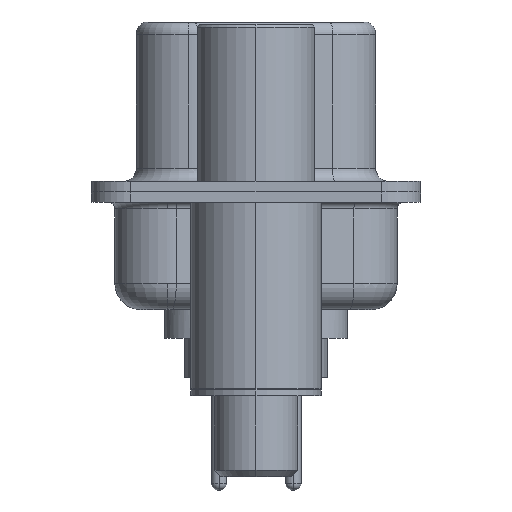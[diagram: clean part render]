
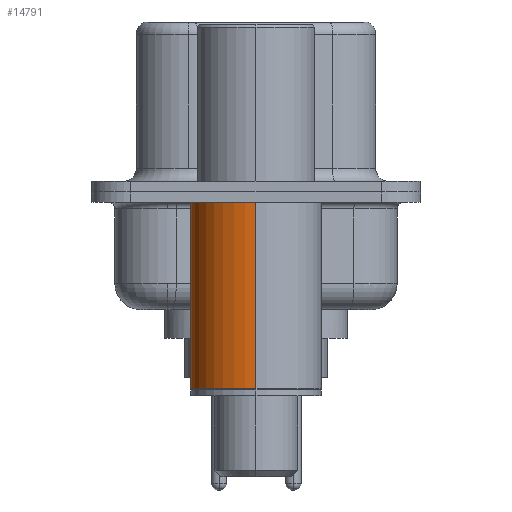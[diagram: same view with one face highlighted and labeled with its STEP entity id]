
A CAD part, left-side view. The second image highlights one B-rep face of the part: STEP entity #14791.
In plain terms, the highlighted cylindrical face has radius 2.5 mm (diameter 5 mm), a partial arc.
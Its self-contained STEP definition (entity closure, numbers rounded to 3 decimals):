
#1159 = EDGE_CURVE ( 'NONE', #7783, #21015, #15888, .T. ) ;
#2001 = DIRECTION ( 'NONE',  ( 0., 0., 1. ) ) ;
#2434 = AXIS2_PLACEMENT_3D ( 'NONE', #13179, #2001, #15097 ) ;
#7620 = DIRECTION ( 'NONE',  ( 1., 0., 0. ) ) ;
#7783 = VERTEX_POINT ( 'NONE', #15548 ) ;
#8595 = CARTESIAN_POINT ( 'NONE',  ( -2.5, 0., -0.4 ) ) ;
#8681 = FACE_OUTER_BOUND ( 'NONE', #11398, .T. ) ;
#8783 = EDGE_CURVE ( 'NONE', #21015, #13180, #20556, .T. ) ;
#9570 = EDGE_CURVE ( 'NONE', #12052, #13180, #22918, .T. ) ;
#10222 = ORIENTED_EDGE ( 'NONE', *, *, #8783, .F. ) ;
#10861 = VECTOR ( 'NONE', #14720, 1000. ) ;
#11142 = DIRECTION ( 'NONE',  ( 0., 0., 1. ) ) ;
#11398 = EDGE_LOOP ( 'NONE', ( #20357, #17075, #10222, #19577 ) ) ;
#11399 = CARTESIAN_POINT ( 'NONE',  ( -2.5, 0., -7.525 ) ) ;
#12052 = VERTEX_POINT ( 'NONE', #11399 ) ;
#12962 = VECTOR ( 'NONE', #20549, 1000. ) ;
#13093 = DIRECTION ( 'NONE',  ( 0., 0., 1. ) ) ;
#13179 = CARTESIAN_POINT ( 'NONE',  ( 0., 0., -7.525 ) ) ;
#13180 = VERTEX_POINT ( 'NONE', #8595 ) ;
#14642 = CARTESIAN_POINT ( 'NONE',  ( 2.5, 0., 0.581 ) ) ;
#14720 = DIRECTION ( 'NONE',  ( 0., 0., 1. ) ) ;
#14791 = ADVANCED_FACE ( 'NONE', ( #8681 ), #23015, .T. ) ;
#14832 = AXIS2_PLACEMENT_3D ( 'NONE', #18840, #13093, #7620 ) ;
#15050 = AXIS2_PLACEMENT_3D ( 'NONE', #22352, #11142, #24262 ) ;
#15097 = DIRECTION ( 'NONE',  ( 1., 0., 0. ) ) ;
#15548 = CARTESIAN_POINT ( 'NONE',  ( 2.5, 0., -7.525 ) ) ;
#15888 = LINE ( 'NONE', #14642, #10861 ) ;
#16976 = CARTESIAN_POINT ( 'NONE',  ( -2.5, 0., 0.581 ) ) ;
#17075 = ORIENTED_EDGE ( 'NONE', *, *, #9570, .T. ) ;
#18625 = CIRCLE ( 'NONE', #2434, 2.5 ) ;
#18840 = CARTESIAN_POINT ( 'NONE',  ( 0., 0., 0.581 ) ) ;
#19577 = ORIENTED_EDGE ( 'NONE', *, *, #1159, .F. ) ;
#20357 = ORIENTED_EDGE ( 'NONE', *, *, #23388, .T. ) ;
#20549 = DIRECTION ( 'NONE',  ( 0., 0., 1. ) ) ;
#20556 = CIRCLE ( 'NONE', #15050, 2.5 ) ;
#21015 = VERTEX_POINT ( 'NONE', #23736 ) ;
#22352 = CARTESIAN_POINT ( 'NONE',  ( 0., 0., -0.4 ) ) ;
#22918 = LINE ( 'NONE', #16976, #12962 ) ;
#23015 = CYLINDRICAL_SURFACE ( 'NONE', #14832, 2.5 ) ;
#23388 = EDGE_CURVE ( 'NONE', #7783, #12052, #18625, .T. ) ;
#23736 = CARTESIAN_POINT ( 'NONE',  ( 2.5, 0., -0.4 ) ) ;
#24262 = DIRECTION ( 'NONE',  ( 1., 0., 0. ) ) ;
